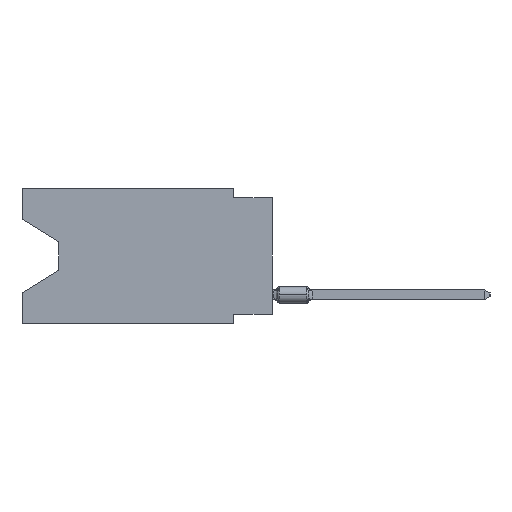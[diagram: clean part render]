
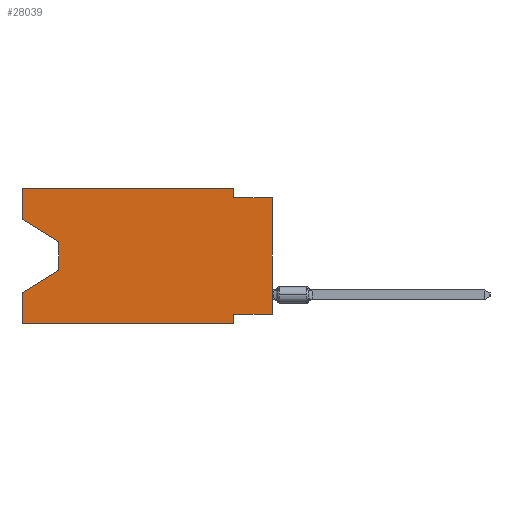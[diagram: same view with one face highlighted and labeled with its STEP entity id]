
A CAD part, left-side view. The second image highlights one B-rep face of the part: STEP entity #28039.
In plain terms, the highlighted planar face has unit normal (-1, 0, 0).
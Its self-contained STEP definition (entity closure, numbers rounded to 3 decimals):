
#164 = LINE ( 'NONE', #3399, #20421 ) ;
#196 = LINE ( 'NONE', #19976, #31293 ) ;
#299 = DIRECTION ( 'NONE',  ( 0., -1., 0. ) ) ;
#501 = CARTESIAN_POINT ( 'NONE',  ( 0., 16.383, 0. ) ) ;
#925 = CARTESIAN_POINT ( 'NONE',  ( 0., 16.383, 0. ) ) ;
#985 = DIRECTION ( 'NONE',  ( 0., 0., -1. ) ) ;
#1040 = DIRECTION ( 'NONE',  ( 0., 0., 1. ) ) ;
#1304 = VECTOR ( 'NONE', #28436, 1000. ) ;
#1453 = VERTEX_POINT ( 'NONE', #7804 ) ;
#1472 = CARTESIAN_POINT ( 'NONE',  ( 0., 16.383, -6.852 ) ) ;
#1772 = VERTEX_POINT ( 'NONE', #30609 ) ;
#1889 = DIRECTION ( 'NONE',  ( 0., 0., -1. ) ) ;
#2308 = VECTOR ( 'NONE', #19628, 1000. ) ;
#2776 = FACE_OUTER_BOUND ( 'NONE', #16866, .T. ) ;
#3399 = CARTESIAN_POINT ( 'NONE',  ( 0., 16.383, 0. ) ) ;
#3548 = CARTESIAN_POINT ( 'NONE',  ( 0., 16.383, -8.89 ) ) ;
#3587 = DIRECTION ( 'NONE',  ( 0., 0.855, -0.519 ) ) ;
#3608 = EDGE_CURVE ( 'NONE', #18338, #16871, #8789, .T. ) ;
#4222 = CARTESIAN_POINT ( 'NONE',  ( 0., 0., -8.255 ) ) ;
#5269 = CARTESIAN_POINT ( 'NONE',  ( 0., 2.54, 0. ) ) ;
#5915 = VECTOR ( 'NONE', #25626, 1000. ) ;
#5938 = CARTESIAN_POINT ( 'NONE',  ( 0., 0., 0. ) ) ;
#6973 = LINE ( 'NONE', #23857, #2308 ) ;
#7561 = ORIENTED_EDGE ( 'NONE', *, *, #17939, .F. ) ;
#7745 = EDGE_CURVE ( 'NONE', #18681, #25482, #23441, .T. ) ;
#7804 = CARTESIAN_POINT ( 'NONE',  ( 0., 16.383, -2.038 ) ) ;
#8026 = CARTESIAN_POINT ( 'NONE',  ( 0., 13.97, -3.505 ) ) ;
#8273 = PLANE ( 'NONE',  #20828 ) ;
#8546 = VERTEX_POINT ( 'NONE', #11997 ) ;
#8738 = ORIENTED_EDGE ( 'NONE', *, *, #21346, .F. ) ;
#8789 = LINE ( 'NONE', #13527, #9920 ) ;
#9256 = EDGE_CURVE ( 'NONE', #8546, #16933, #18886, .T. ) ;
#9543 = VECTOR ( 'NONE', #29330, 1000. ) ;
#9920 = VECTOR ( 'NONE', #1040, 1000. ) ;
#10090 = DIRECTION ( 'NONE',  ( 0., -0.855, -0.519 ) ) ;
#10094 = CARTESIAN_POINT ( 'NONE',  ( 0., 13.97, -5.385 ) ) ;
#10292 = DIRECTION ( 'NONE',  ( 0., 0., -1. ) ) ;
#10375 = CARTESIAN_POINT ( 'NONE',  ( 0., 2.54, -8.89 ) ) ;
#11997 = CARTESIAN_POINT ( 'NONE',  ( 0., 0., -8.255 ) ) ;
#12179 = LINE ( 'NONE', #10375, #24722 ) ;
#12985 = CARTESIAN_POINT ( 'NONE',  ( 0., 16.383, -8.89 ) ) ;
#13210 = LINE ( 'NONE', #23094, #14246 ) ;
#13527 = CARTESIAN_POINT ( 'NONE',  ( 0., 16.383, 0. ) ) ;
#13710 = VECTOR ( 'NONE', #3587, 1000. ) ;
#13906 = ORIENTED_EDGE ( 'NONE', *, *, #14230, .F. ) ;
#14230 = EDGE_CURVE ( 'NONE', #1772, #14977, #12179, .T. ) ;
#14246 = VECTOR ( 'NONE', #10292, 1000. ) ;
#14931 = ORIENTED_EDGE ( 'NONE', *, *, #17969, .F. ) ;
#14977 = VERTEX_POINT ( 'NONE', #16163 ) ;
#14988 = CARTESIAN_POINT ( 'NONE',  ( 0., 13.97, -3.505 ) ) ;
#15570 = ORIENTED_EDGE ( 'NONE', *, *, #7745, .F. ) ;
#15699 = ORIENTED_EDGE ( 'NONE', *, *, #3608, .F. ) ;
#15758 = ORIENTED_EDGE ( 'NONE', *, *, #25089, .F. ) ;
#15921 = LINE ( 'NONE', #25811, #13710 ) ;
#16163 = CARTESIAN_POINT ( 'NONE',  ( 0., 2.54, -8.89 ) ) ;
#16866 = EDGE_LOOP ( 'NONE', ( #26114, #29973, #23996, #15699, #31899, #13906, #7561, #28692, #14931, #8738, #15570, #15758 ) ) ;
#16871 = VERTEX_POINT ( 'NONE', #1472 ) ;
#16933 = VERTEX_POINT ( 'NONE', #19777 ) ;
#17519 = VECTOR ( 'NONE', #1889, 1000. ) ;
#17755 = EDGE_CURVE ( 'NONE', #1453, #29870, #196, .T. ) ;
#17913 = EDGE_CURVE ( 'NONE', #21768, #16871, #15921, .T. ) ;
#17939 = EDGE_CURVE ( 'NONE', #8546, #1772, #28373, .T. ) ;
#17969 = EDGE_CURVE ( 'NONE', #30361, #16933, #6973, .T. ) ;
#18338 = VERTEX_POINT ( 'NONE', #3548 ) ;
#18681 = VERTEX_POINT ( 'NONE', #925 ) ;
#18886 = LINE ( 'NONE', #5938, #1304 ) ;
#19628 = DIRECTION ( 'NONE',  ( 0., -1., 0. ) ) ;
#19777 = CARTESIAN_POINT ( 'NONE',  ( 0., 0., -0.635 ) ) ;
#19976 = CARTESIAN_POINT ( 'NONE',  ( 0., 16.383, -2.038 ) ) ;
#20421 = VECTOR ( 'NONE', #25135, 1000. ) ;
#20691 = CARTESIAN_POINT ( 'NONE',  ( 0., 16.383, 0. ) ) ;
#20828 = AXIS2_PLACEMENT_3D ( 'NONE', #501, #29829, #985 ) ;
#21346 = EDGE_CURVE ( 'NONE', #25482, #30361, #13210, .T. ) ;
#21768 = VERTEX_POINT ( 'NONE', #10094 ) ;
#23094 = CARTESIAN_POINT ( 'NONE',  ( 0., 2.54, 0. ) ) ;
#23441 = LINE ( 'NONE', #20691, #24017 ) ;
#23857 = CARTESIAN_POINT ( 'NONE',  ( 0., 0., -0.635 ) ) ;
#23996 = ORIENTED_EDGE ( 'NONE', *, *, #17913, .T. ) ;
#24017 = VECTOR ( 'NONE', #299, 1000. ) ;
#24722 = VECTOR ( 'NONE', #30132, 1000. ) ;
#25089 = EDGE_CURVE ( 'NONE', #1453, #18681, #164, .T. ) ;
#25135 = DIRECTION ( 'NONE',  ( 0., 0., 1. ) ) ;
#25482 = VERTEX_POINT ( 'NONE', #5269 ) ;
#25626 = DIRECTION ( 'NONE',  ( 0., -1., 0. ) ) ;
#25811 = CARTESIAN_POINT ( 'NONE',  ( 0., 13.97, -5.385 ) ) ;
#26114 = ORIENTED_EDGE ( 'NONE', *, *, #17755, .T. ) ;
#26379 = EDGE_CURVE ( 'NONE', #18338, #14977, #30461, .T. ) ;
#28039 = ADVANCED_FACE ( 'NONE', ( #2776 ), #8273, .F. ) ;
#28373 = LINE ( 'NONE', #4222, #9543 ) ;
#28436 = DIRECTION ( 'NONE',  ( 0., 0., 1. ) ) ;
#28677 = EDGE_CURVE ( 'NONE', #29870, #21768, #29112, .T. ) ;
#28692 = ORIENTED_EDGE ( 'NONE', *, *, #9256, .T. ) ;
#29112 = LINE ( 'NONE', #14988, #17519 ) ;
#29330 = DIRECTION ( 'NONE',  ( 0., 1., 0. ) ) ;
#29829 = DIRECTION ( 'NONE',  ( 1., 0., 0. ) ) ;
#29870 = VERTEX_POINT ( 'NONE', #8026 ) ;
#29973 = ORIENTED_EDGE ( 'NONE', *, *, #28677, .T. ) ;
#30132 = DIRECTION ( 'NONE',  ( 0., 0., -1. ) ) ;
#30356 = CARTESIAN_POINT ( 'NONE',  ( 0., 2.54, -0.635 ) ) ;
#30361 = VERTEX_POINT ( 'NONE', #30356 ) ;
#30461 = LINE ( 'NONE', #12985, #5915 ) ;
#30609 = CARTESIAN_POINT ( 'NONE',  ( 0., 2.54, -8.255 ) ) ;
#31293 = VECTOR ( 'NONE', #10090, 1000. ) ;
#31899 = ORIENTED_EDGE ( 'NONE', *, *, #26379, .T. ) ;
